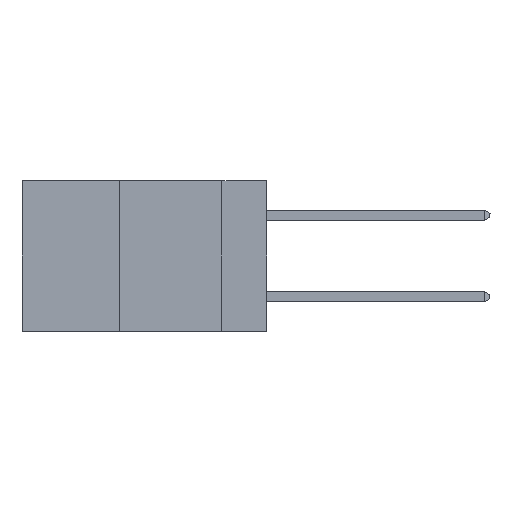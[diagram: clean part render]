
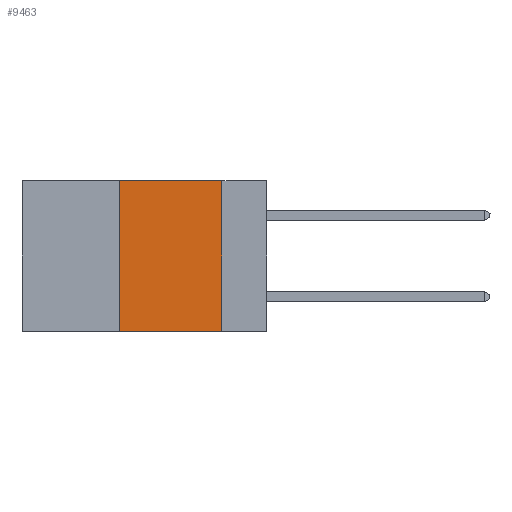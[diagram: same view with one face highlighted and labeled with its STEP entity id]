
A CAD part, left-side view. The second image highlights one B-rep face of the part: STEP entity #9463.
In plain terms, the highlighted planar face has unit normal (-1, 0, 0).
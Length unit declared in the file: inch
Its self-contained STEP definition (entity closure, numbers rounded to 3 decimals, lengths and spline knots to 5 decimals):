
#251 = CARTESIAN_POINT ( 'NONE',  ( 0., 0.6, 0. ) ) ;
#600 = VERTEX_POINT ( 'NONE', #16692 ) ;
#1900 = LINE ( 'NONE', #13171, #20700 ) ;
#1971 = DIRECTION ( 'NONE',  ( 0., -1., 0. ) ) ;
#2338 = FACE_OUTER_BOUND ( 'NONE', #18057, .T. ) ;
#3347 = VERTEX_POINT ( 'NONE', #10879 ) ;
#3539 = PLANE ( 'NONE',  #15525 ) ;
#5251 = DIRECTION ( 'NONE',  ( 0., 0., -1. ) ) ;
#5979 = ORIENTED_EDGE ( 'NONE', *, *, #14693, .F. ) ;
#6034 = CARTESIAN_POINT ( 'NONE',  ( 0., 0.11, -0.37 ) ) ;
#6199 = EDGE_CURVE ( 'NONE', #14412, #3347, #14699, .T. ) ;
#6808 = LINE ( 'NONE', #251, #16812 ) ;
#7140 = CARTESIAN_POINT ( 'NONE',  ( 0., 0.36, -0.37 ) ) ;
#7991 = DIRECTION ( 'NONE',  ( 0., 0., -1. ) ) ;
#8069 = DIRECTION ( 'NONE',  ( 0., 0., 1. ) ) ;
#8193 = ORIENTED_EDGE ( 'NONE', *, *, #18699, .T. ) ;
#8703 = VECTOR ( 'NONE', #8069, 39.37008 ) ;
#9185 = VERTEX_POINT ( 'NONE', #6034 ) ;
#9463 = ADVANCED_FACE ( 'NONE', ( #2338 ), #3539, .F. ) ;
#10879 = CARTESIAN_POINT ( 'NONE',  ( 0., 0.36, 0. ) ) ;
#11328 = ORIENTED_EDGE ( 'NONE', *, *, #6199, .F. ) ;
#11775 = CARTESIAN_POINT ( 'NONE',  ( 0., 0.6, 0. ) ) ;
#11876 = ORIENTED_EDGE ( 'NONE', *, *, #14850, .F. ) ;
#12813 = CARTESIAN_POINT ( 'NONE',  ( 0., 0.11, 0. ) ) ;
#12997 = CARTESIAN_POINT ( 'NONE',  ( 0., 0.36, 0. ) ) ;
#13059 = DIRECTION ( 'NONE',  ( 0., -1., 0. ) ) ;
#13171 = CARTESIAN_POINT ( 'NONE',  ( 0., 0.6, -0.37 ) ) ;
#13384 = DIRECTION ( 'NONE',  ( 1., 0., 0. ) ) ;
#14412 = VERTEX_POINT ( 'NONE', #7140 ) ;
#14693 = EDGE_CURVE ( 'NONE', #600, #9185, #17851, .T. ) ;
#14699 = LINE ( 'NONE', #12997, #8703 ) ;
#14850 = EDGE_CURVE ( 'NONE', #3347, #600, #6808, .T. ) ;
#15525 = AXIS2_PLACEMENT_3D ( 'NONE', #11775, #13384, #5251 ) ;
#16692 = CARTESIAN_POINT ( 'NONE',  ( 0., 0.11, 0. ) ) ;
#16812 = VECTOR ( 'NONE', #1971, 39.37008 ) ;
#17480 = VECTOR ( 'NONE', #7991, 39.37008 ) ;
#17851 = LINE ( 'NONE', #12813, #17480 ) ;
#18057 = EDGE_LOOP ( 'NONE', ( #5979, #11876, #11328, #8193 ) ) ;
#18699 = EDGE_CURVE ( 'NONE', #14412, #9185, #1900, .T. ) ;
#20700 = VECTOR ( 'NONE', #13059, 39.37008 ) ;
